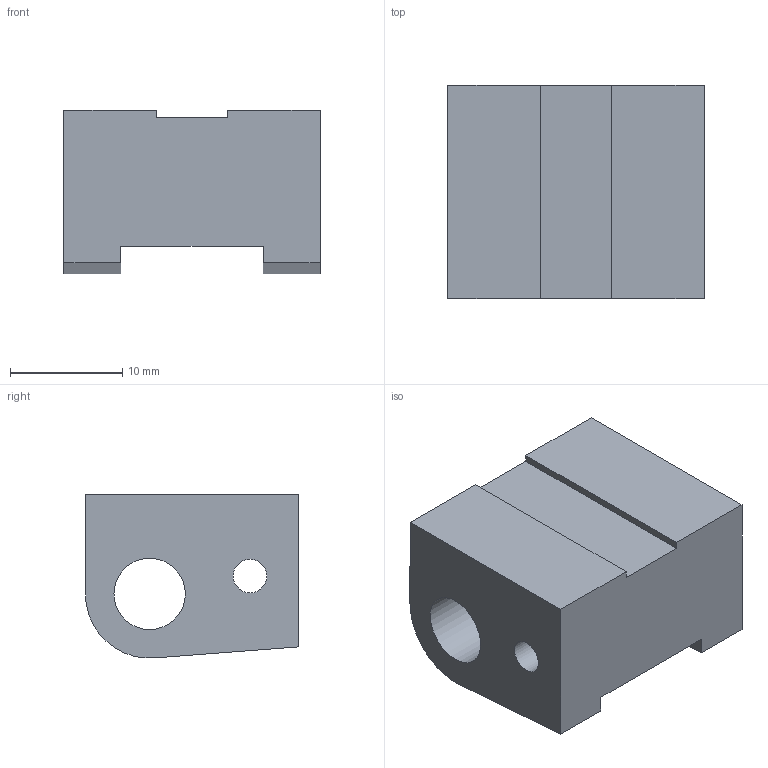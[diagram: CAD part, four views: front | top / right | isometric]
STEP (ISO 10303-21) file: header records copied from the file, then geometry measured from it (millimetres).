
FILE_DESCRIPTION (( 'STEP AP214' ), '1' );
FILE_NAME ('Phobos_Mag_Well_Front.step', '2016-01-30T20:06:17', ( 'WarFairy' ), ( '' ), 'SwSTEP 2.0', 'SolidWorks 2015', '' );
FILE_SCHEMA (( 'AUTOMOTIVE_DESIGN' ));
Length unit declared in the file: millimetre
Products named in the file (1): Phobos_Mag_Well_Front
Bounding box: 22.81 x 18.98 x 14.59 mm (x, y, z)
Volume: 3523.7 mm3; surface area: 2557.2 mm2
Topology: 1 solids, 1 shells, 21 faces, 59 edges, 40 vertices
Faces by surface type: plane 16, cylinder 5
Full cylindrical faces by diameter (mm): 3 x1, 6.35 x2
Entity records: 692 total; most frequent: CARTESIAN_POINT 114, DIRECTION 108, ORIENTED_EDGE 108, EDGE_CURVE 54, VECTOR 44, LINE 44, VERTEX_POINT 38, AXIS2_PLACEMENT_3D 32
